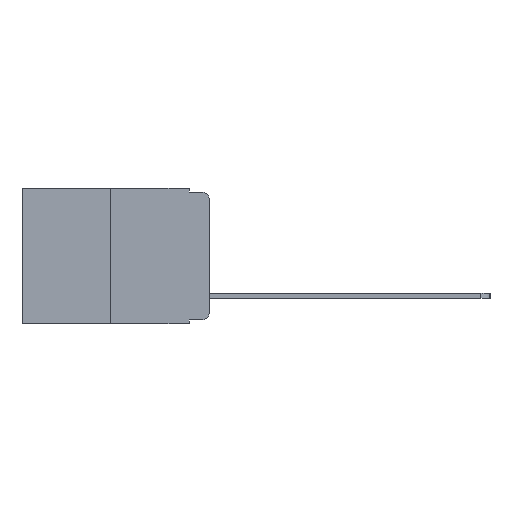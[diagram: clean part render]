
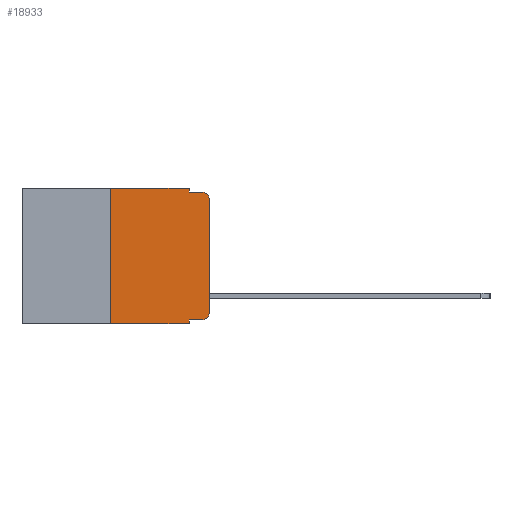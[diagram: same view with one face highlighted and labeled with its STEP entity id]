
A CAD part, left-side view. The second image highlights one B-rep face of the part: STEP entity #18933.
In plain terms, the highlighted planar face has unit normal (-1, 0, 0).
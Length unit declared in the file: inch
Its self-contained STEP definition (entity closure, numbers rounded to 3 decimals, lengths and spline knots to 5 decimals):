
#166 = DIRECTION ( 'NONE',  ( 0., 0., -1. ) ) ;
#651 = VERTEX_POINT ( 'NONE', #8844 ) ;
#911 = CARTESIAN_POINT ( 'NONE',  ( 0., 0.051, -0.333 ) ) ;
#1371 = ORIENTED_EDGE ( 'NONE', *, *, #11673, .T. ) ;
#1587 = CARTESIAN_POINT ( 'NONE',  ( 0., 0.25, 0. ) ) ;
#2439 = VERTEX_POINT ( 'NONE', #3301 ) ;
#2643 = CARTESIAN_POINT ( 'NONE',  ( 0., 0.051, 0. ) ) ;
#2902 = LINE ( 'NONE', #1587, #17048 ) ;
#2927 = CARTESIAN_POINT ( 'NONE',  ( 0., 0.473, 0. ) ) ;
#3016 = ORIENTED_EDGE ( 'NONE', *, *, #20494, .T. ) ;
#3040 = ORIENTED_EDGE ( 'NONE', *, *, #8935, .T. ) ;
#3301 = CARTESIAN_POINT ( 'NONE',  ( 0., 0.051, -0.01 ) ) ;
#3541 = DIRECTION ( 'NONE',  ( 0., 0., 1. ) ) ;
#3679 = EDGE_CURVE ( 'NONE', #18925, #22278, #9982, .T. ) ;
#3787 = LINE ( 'NONE', #7874, #8753 ) ;
#4105 = LINE ( 'NONE', #19066, #18121 ) ;
#4398 = LINE ( 'NONE', #23666, #23667 ) ;
#4415 = VECTOR ( 'NONE', #8425, 39.37008 ) ;
#4672 = CARTESIAN_POINT ( 'NONE',  ( 0., 0.473, 0. ) ) ;
#4866 = CARTESIAN_POINT ( 'NONE',  ( 0., 0., -0.03 ) ) ;
#5217 = PLANE ( 'NONE',  #5827 ) ;
#5827 = AXIS2_PLACEMENT_3D ( 'NONE', #2927, #18021, #7101 ) ;
#5856 = CIRCLE ( 'NONE', #16911, 0.02 ) ;
#5992 = VERTEX_POINT ( 'NONE', #14341 ) ;
#6790 = EDGE_CURVE ( 'NONE', #12064, #20882, #12362, .T. ) ;
#7010 = VECTOR ( 'NONE', #22241, 39.37008 ) ;
#7101 = DIRECTION ( 'NONE',  ( 0., 0., -1. ) ) ;
#7371 = VECTOR ( 'NONE', #18391, 39.37008 ) ;
#7589 = LINE ( 'NONE', #13405, #7010 ) ;
#7874 = CARTESIAN_POINT ( 'NONE',  ( 0., 0.051, 0. ) ) ;
#7888 = VERTEX_POINT ( 'NONE', #911 ) ;
#7893 = VECTOR ( 'NONE', #21673, 39.37008 ) ;
#8425 = DIRECTION ( 'NONE',  ( 0., -1., 0. ) ) ;
#8753 = VECTOR ( 'NONE', #9772, 39.37008 ) ;
#8844 = CARTESIAN_POINT ( 'NONE',  ( 0., 0., -0.313 ) ) ;
#8935 = EDGE_CURVE ( 'NONE', #651, #15386, #7589, .T. ) ;
#8973 = EDGE_CURVE ( 'NONE', #15386, #5992, #5856, .T. ) ;
#9042 = EDGE_CURVE ( 'NONE', #2439, #5992, #4105, .T. ) ;
#9081 = EDGE_CURVE ( 'NONE', #22278, #2439, #12830, .T. ) ;
#9088 = EDGE_CURVE ( 'NONE', #12064, #18925, #2902, .T. ) ;
#9262 = EDGE_CURVE ( 'NONE', #7888, #20882, #3787, .T. ) ;
#9772 = DIRECTION ( 'NONE',  ( 0., 0., -1. ) ) ;
#9827 = EDGE_LOOP ( 'NONE', ( #3040, #16918, #17451, #23257, #15803, #22464, #22826, #20322, #1371, #3016 ) ) ;
#9946 = CARTESIAN_POINT ( 'NONE',  ( 0., 0.02, -0.03 ) ) ;
#9982 = LINE ( 'NONE', #4672, #4415 ) ;
#10526 = CARTESIAN_POINT ( 'NONE',  ( 0., 0.25, -0.343 ) ) ;
#10824 = CIRCLE ( 'NONE', #23419, 0.02 ) ;
#11463 = DIRECTION ( 'NONE',  ( -1., 0., 0. ) ) ;
#11673 = EDGE_CURVE ( 'NONE', #7888, #11687, #4398, .T. ) ;
#11687 = VERTEX_POINT ( 'NONE', #14840 ) ;
#11822 = DIRECTION ( 'NONE',  ( 0., 0., -1. ) ) ;
#12064 = VERTEX_POINT ( 'NONE', #10526 ) ;
#12315 = CARTESIAN_POINT ( 'NONE',  ( 0., 0.051, 0. ) ) ;
#12362 = LINE ( 'NONE', #23651, #7371 ) ;
#12830 = LINE ( 'NONE', #2643, #7893 ) ;
#13042 = DIRECTION ( 'NONE',  ( 0., -1., 0. ) ) ;
#13405 = CARTESIAN_POINT ( 'NONE',  ( 0., 0., 0. ) ) ;
#14341 = CARTESIAN_POINT ( 'NONE',  ( 0., 0.02, -0.01 ) ) ;
#14453 = CARTESIAN_POINT ( 'NONE',  ( 0., 0.25, 0. ) ) ;
#14840 = CARTESIAN_POINT ( 'NONE',  ( 0., 0.02, -0.333 ) ) ;
#15386 = VERTEX_POINT ( 'NONE', #4866 ) ;
#15580 = DIRECTION ( 'NONE',  ( 0., -1., 0. ) ) ;
#15803 = ORIENTED_EDGE ( 'NONE', *, *, #3679, .F. ) ;
#16911 = AXIS2_PLACEMENT_3D ( 'NONE', #9946, #22480, #11822 ) ;
#16918 = ORIENTED_EDGE ( 'NONE', *, *, #8973, .T. ) ;
#17048 = VECTOR ( 'NONE', #3541, 39.37008 ) ;
#17451 = ORIENTED_EDGE ( 'NONE', *, *, #9042, .F. ) ;
#17933 = FACE_OUTER_BOUND ( 'NONE', #9827, .T. ) ;
#18016 = CARTESIAN_POINT ( 'NONE',  ( 0., 0.051, -0.343 ) ) ;
#18021 = DIRECTION ( 'NONE',  ( 1., 0., 0. ) ) ;
#18121 = VECTOR ( 'NONE', #15580, 39.37008 ) ;
#18391 = DIRECTION ( 'NONE',  ( 0., -1., 0. ) ) ;
#18925 = VERTEX_POINT ( 'NONE', #14453 ) ;
#18933 = ADVANCED_FACE ( 'NONE', ( #17933 ), #5217, .F. ) ;
#19066 = CARTESIAN_POINT ( 'NONE',  ( 0., 0.051, -0.01 ) ) ;
#20322 = ORIENTED_EDGE ( 'NONE', *, *, #9262, .F. ) ;
#20494 = EDGE_CURVE ( 'NONE', #11687, #651, #10824, .T. ) ;
#20882 = VERTEX_POINT ( 'NONE', #18016 ) ;
#21673 = DIRECTION ( 'NONE',  ( 0., 0., -1. ) ) ;
#22143 = CARTESIAN_POINT ( 'NONE',  ( 0., 0.02, -0.313 ) ) ;
#22241 = DIRECTION ( 'NONE',  ( 0., 0., 1. ) ) ;
#22278 = VERTEX_POINT ( 'NONE', #12315 ) ;
#22464 = ORIENTED_EDGE ( 'NONE', *, *, #9088, .F. ) ;
#22480 = DIRECTION ( 'NONE',  ( -1., 0., 0. ) ) ;
#22826 = ORIENTED_EDGE ( 'NONE', *, *, #6790, .T. ) ;
#23257 = ORIENTED_EDGE ( 'NONE', *, *, #9081, .F. ) ;
#23419 = AXIS2_PLACEMENT_3D ( 'NONE', #22143, #11463, #166 ) ;
#23651 = CARTESIAN_POINT ( 'NONE',  ( 0., 0.473, -0.343 ) ) ;
#23666 = CARTESIAN_POINT ( 'NONE',  ( 0., 0.051, -0.333 ) ) ;
#23667 = VECTOR ( 'NONE', #13042, 39.37008 ) ;
